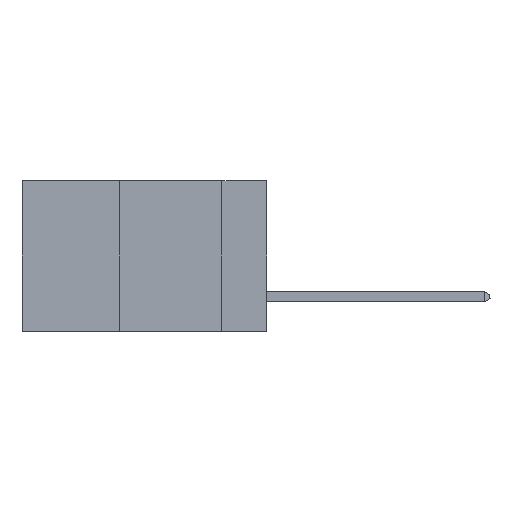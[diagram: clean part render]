
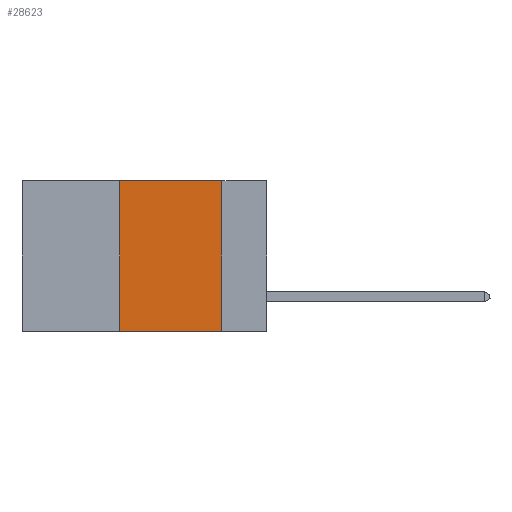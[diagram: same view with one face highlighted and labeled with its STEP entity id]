
A CAD part, left-side view. The second image highlights one B-rep face of the part: STEP entity #28623.
In plain terms, the highlighted planar face has unit normal (-1, 0, 0).
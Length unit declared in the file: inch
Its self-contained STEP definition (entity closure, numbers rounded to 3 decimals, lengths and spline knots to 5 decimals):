
#165 = EDGE_CURVE ( 'NONE', #9497, #29050, #919, .T. ) ;
#919 = LINE ( 'NONE', #2553, #34172 ) ;
#1401 = ORIENTED_EDGE ( 'NONE', *, *, #24617, .F. ) ;
#1791 = DIRECTION ( 'NONE',  ( 0., 0., -1. ) ) ;
#2553 = CARTESIAN_POINT ( 'NONE',  ( 0., 0.6, -0.37 ) ) ;
#2726 = LINE ( 'NONE', #11723, #34912 ) ;
#2840 = VERTEX_POINT ( 'NONE', #6601 ) ;
#3489 = CARTESIAN_POINT ( 'NONE',  ( 0., 0.6, 0. ) ) ;
#4562 = CARTESIAN_POINT ( 'NONE',  ( 0., 0.11, 0. ) ) ;
#6601 = CARTESIAN_POINT ( 'NONE',  ( 0., 0.11, 0. ) ) ;
#6993 = EDGE_CURVE ( 'NONE', #2840, #29050, #38536, .T. ) ;
#9497 = VERTEX_POINT ( 'NONE', #34738 ) ;
#11723 = CARTESIAN_POINT ( 'NONE',  ( 0., 0.6, 0. ) ) ;
#11867 = DIRECTION ( 'NONE',  ( 0., -1., 0. ) ) ;
#16439 = CARTESIAN_POINT ( 'NONE',  ( 0., 0.36, 0. ) ) ;
#17441 = ORIENTED_EDGE ( 'NONE', *, *, #6993, .F. ) ;
#21300 = CARTESIAN_POINT ( 'NONE',  ( 0., 0.11, -0.37 ) ) ;
#21935 = LINE ( 'NONE', #31031, #30456 ) ;
#22665 = DIRECTION ( 'NONE',  ( 1., 0., 0. ) ) ;
#24617 = EDGE_CURVE ( 'NONE', #9497, #38111, #21935, .T. ) ;
#25093 = DIRECTION ( 'NONE',  ( 0., -1., 0. ) ) ;
#26567 = ORIENTED_EDGE ( 'NONE', *, *, #31141, .F. ) ;
#28623 = ADVANCED_FACE ( 'NONE', ( #28686 ), #41638, .F. ) ;
#28686 = FACE_OUTER_BOUND ( 'NONE', #36167, .T. ) ;
#29050 = VERTEX_POINT ( 'NONE', #21300 ) ;
#29269 = DIRECTION ( 'NONE',  ( 0., 0., -1. ) ) ;
#30456 = VECTOR ( 'NONE', #37466, 39.37008 ) ;
#31031 = CARTESIAN_POINT ( 'NONE',  ( 0., 0.36, 0. ) ) ;
#31141 = EDGE_CURVE ( 'NONE', #38111, #2840, #2726, .T. ) ;
#34172 = VECTOR ( 'NONE', #25093, 39.37008 ) ;
#34738 = CARTESIAN_POINT ( 'NONE',  ( 0., 0.36, -0.37 ) ) ;
#34912 = VECTOR ( 'NONE', #11867, 39.37008 ) ;
#35871 = AXIS2_PLACEMENT_3D ( 'NONE', #3489, #22665, #29269 ) ;
#36016 = VECTOR ( 'NONE', #1791, 39.37008 ) ;
#36167 = EDGE_LOOP ( 'NONE', ( #17441, #26567, #1401, #39037 ) ) ;
#37466 = DIRECTION ( 'NONE',  ( 0., 0., 1. ) ) ;
#38111 = VERTEX_POINT ( 'NONE', #16439 ) ;
#38536 = LINE ( 'NONE', #4562, #36016 ) ;
#39037 = ORIENTED_EDGE ( 'NONE', *, *, #165, .T. ) ;
#41638 = PLANE ( 'NONE',  #35871 ) ;
